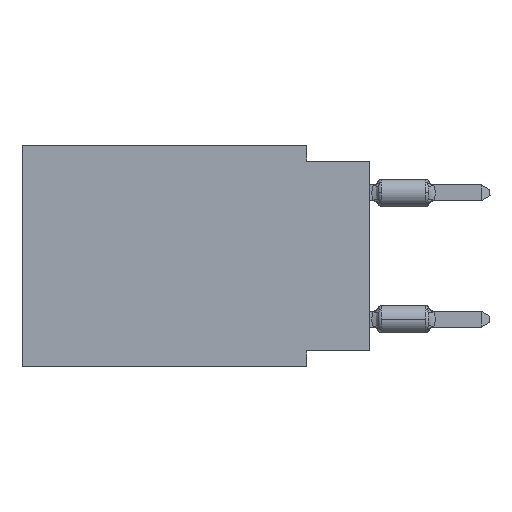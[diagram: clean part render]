
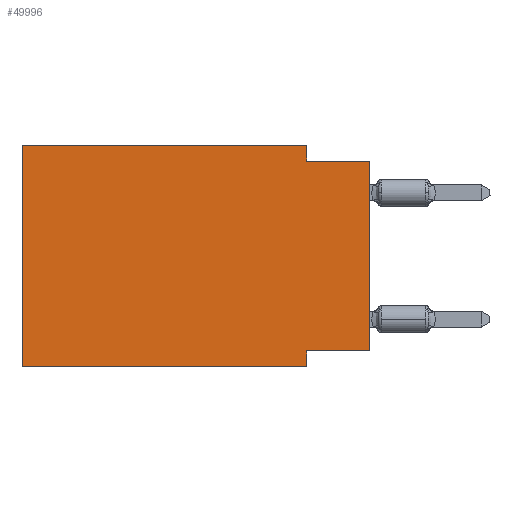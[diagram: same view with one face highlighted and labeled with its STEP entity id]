
A CAD part, left-side view. The second image highlights one B-rep face of the part: STEP entity #49996.
In plain terms, the highlighted planar face has unit normal (-1, 0, 0).
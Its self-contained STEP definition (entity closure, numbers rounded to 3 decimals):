
#861 = CARTESIAN_POINT ( 'NONE',  ( 0., 13.97, 0. ) ) ;
#1478 = EDGE_LOOP ( 'NONE', ( #51326, #4386, #9347, #34866, #16390, #17814, #34790, #19156 ) ) ;
#2489 = DIRECTION ( 'NONE',  ( 0., 0., -1. ) ) ;
#2545 = DIRECTION ( 'NONE',  ( 0., 0., -1. ) ) ;
#4386 = ORIENTED_EDGE ( 'NONE', *, *, #29237, .F. ) ;
#6527 = FACE_OUTER_BOUND ( 'NONE', #1478, .T. ) ;
#7256 = EDGE_CURVE ( 'NONE', #50607, #10537, #9848, .T. ) ;
#7520 = DIRECTION ( 'NONE',  ( 0., 0., 1. ) ) ;
#7579 = CARTESIAN_POINT ( 'NONE',  ( 0., 13.97, 0. ) ) ;
#7833 = DIRECTION ( 'NONE',  ( 0., -1., 0. ) ) ;
#8556 = CARTESIAN_POINT ( 'NONE',  ( 0., 13.97, -8.89 ) ) ;
#9347 = ORIENTED_EDGE ( 'NONE', *, *, #50483, .F. ) ;
#9848 = LINE ( 'NONE', #34519, #17646 ) ;
#10537 = VERTEX_POINT ( 'NONE', #39249 ) ;
#10763 = DIRECTION ( 'NONE',  ( 1., 0., 0. ) ) ;
#11292 = CARTESIAN_POINT ( 'NONE',  ( 0., 13.97, 0. ) ) ;
#11310 = DIRECTION ( 'NONE',  ( 0., 0., 1. ) ) ;
#11514 = CARTESIAN_POINT ( 'NONE',  ( 0., 2.54, -0.635 ) ) ;
#12383 = DIRECTION ( 'NONE',  ( 0., 0., -1. ) ) ;
#12592 = LINE ( 'NONE', #7579, #45541 ) ;
#13423 = CARTESIAN_POINT ( 'NONE',  ( 0., 2.54, -8.89 ) ) ;
#15206 = EDGE_CURVE ( 'NONE', #18766, #51788, #23454, .T. ) ;
#15657 = AXIS2_PLACEMENT_3D ( 'NONE', #11292, #10763, #2545 ) ;
#15886 = VERTEX_POINT ( 'NONE', #22259 ) ;
#16390 = ORIENTED_EDGE ( 'NONE', *, *, #15206, .F. ) ;
#17646 = VECTOR ( 'NONE', #22054, 1000. ) ;
#17814 = ORIENTED_EDGE ( 'NONE', *, *, #20378, .T. ) ;
#18766 = VERTEX_POINT ( 'NONE', #47046 ) ;
#19156 = ORIENTED_EDGE ( 'NONE', *, *, #7256, .F. ) ;
#20378 = EDGE_CURVE ( 'NONE', #18766, #15886, #44894, .T. ) ;
#22054 = DIRECTION ( 'NONE',  ( 0., 1., 0. ) ) ;
#22259 = CARTESIAN_POINT ( 'NONE',  ( 0., 2.54, -8.89 ) ) ;
#23259 = LINE ( 'NONE', #26434, #49023 ) ;
#23326 = EDGE_CURVE ( 'NONE', #50607, #42166, #23259, .T. ) ;
#23454 = LINE ( 'NONE', #43864, #49537 ) ;
#23857 = VERTEX_POINT ( 'NONE', #11514 ) ;
#25117 = LINE ( 'NONE', #13423, #27792 ) ;
#25415 = VECTOR ( 'NONE', #34666, 1000. ) ;
#26434 = CARTESIAN_POINT ( 'NONE',  ( 0., 0., 0. ) ) ;
#27792 = VECTOR ( 'NONE', #12383, 1000. ) ;
#29237 = EDGE_CURVE ( 'NONE', #23857, #42166, #30684, .T. ) ;
#30180 = CARTESIAN_POINT ( 'NONE',  ( 0., 0., -0.635 ) ) ;
#30658 = PLANE ( 'NONE',  #15657 ) ;
#30684 = LINE ( 'NONE', #51109, #25415 ) ;
#30865 = LINE ( 'NONE', #38818, #42787 ) ;
#34519 = CARTESIAN_POINT ( 'NONE',  ( 0., 0., -8.255 ) ) ;
#34666 = DIRECTION ( 'NONE',  ( 0., -1., 0. ) ) ;
#34790 = ORIENTED_EDGE ( 'NONE', *, *, #45120, .F. ) ;
#34866 = ORIENTED_EDGE ( 'NONE', *, *, #48802, .F. ) ;
#38818 = CARTESIAN_POINT ( 'NONE',  ( 0., 2.54, 0. ) ) ;
#39249 = CARTESIAN_POINT ( 'NONE',  ( 0., 2.54, -8.255 ) ) ;
#42091 = VERTEX_POINT ( 'NONE', #48245 ) ;
#42166 = VERTEX_POINT ( 'NONE', #30180 ) ;
#42787 = VECTOR ( 'NONE', #2489, 1000. ) ;
#43696 = VECTOR ( 'NONE', #45422, 1000. ) ;
#43864 = CARTESIAN_POINT ( 'NONE',  ( 0., 13.97, 0. ) ) ;
#44628 = CARTESIAN_POINT ( 'NONE',  ( 0., 0., -8.255 ) ) ;
#44894 = LINE ( 'NONE', #8556, #43696 ) ;
#45120 = EDGE_CURVE ( 'NONE', #10537, #15886, #25117, .T. ) ;
#45422 = DIRECTION ( 'NONE',  ( 0., -1., 0. ) ) ;
#45541 = VECTOR ( 'NONE', #7833, 1000. ) ;
#47046 = CARTESIAN_POINT ( 'NONE',  ( 0., 13.97, -8.89 ) ) ;
#48245 = CARTESIAN_POINT ( 'NONE',  ( 0., 2.54, 0. ) ) ;
#48802 = EDGE_CURVE ( 'NONE', #51788, #42091, #12592, .T. ) ;
#49023 = VECTOR ( 'NONE', #11310, 1000. ) ;
#49537 = VECTOR ( 'NONE', #7520, 1000. ) ;
#49996 = ADVANCED_FACE ( 'NONE', ( #6527 ), #30658, .F. ) ;
#50483 = EDGE_CURVE ( 'NONE', #42091, #23857, #30865, .T. ) ;
#50607 = VERTEX_POINT ( 'NONE', #44628 ) ;
#51109 = CARTESIAN_POINT ( 'NONE',  ( 0., 0., -0.635 ) ) ;
#51326 = ORIENTED_EDGE ( 'NONE', *, *, #23326, .T. ) ;
#51788 = VERTEX_POINT ( 'NONE', #861 ) ;
